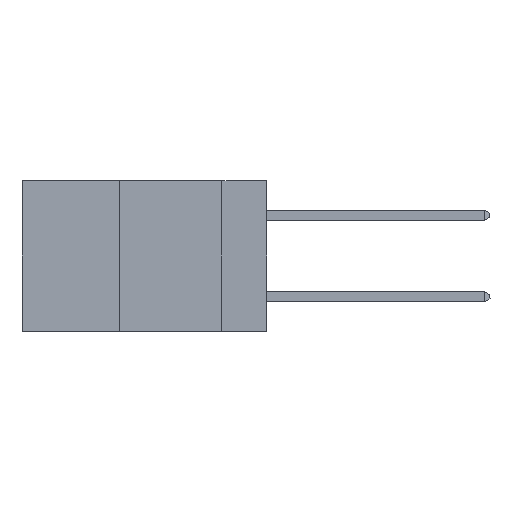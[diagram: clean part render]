
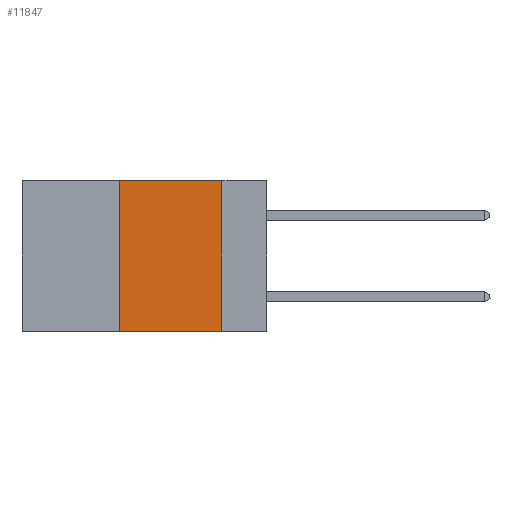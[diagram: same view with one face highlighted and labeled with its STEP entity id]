
A CAD part, left-side view. The second image highlights one B-rep face of the part: STEP entity #11847.
In plain terms, the highlighted planar face has unit normal (-1, 0, 0).
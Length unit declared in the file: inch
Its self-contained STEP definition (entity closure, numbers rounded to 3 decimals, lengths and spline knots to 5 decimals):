
#22 = EDGE_CURVE ( 'NONE', #6171, #15439, #13116, .T. ) ;
#527 = CARTESIAN_POINT ( 'NONE',  ( 0., 0.6, 0. ) ) ;
#677 = VECTOR ( 'NONE', #1669, 39.37008 ) ;
#1466 = DIRECTION ( 'NONE',  ( 1., 0., 0. ) ) ;
#1669 = DIRECTION ( 'NONE',  ( 0., -1., 0. ) ) ;
#1862 = AXIS2_PLACEMENT_3D ( 'NONE', #12660, #1466, #11447 ) ;
#2113 = LINE ( 'NONE', #4818, #7542 ) ;
#3150 = EDGE_LOOP ( 'NONE', ( #13163, #9197, #14579, #9522 ) ) ;
#3250 = VECTOR ( 'NONE', #5093, 39.37008 ) ;
#4285 = EDGE_CURVE ( 'NONE', #4865, #7811, #8316, .T. ) ;
#4818 = CARTESIAN_POINT ( 'NONE',  ( 0., 0.36, 0. ) ) ;
#4865 = VERTEX_POINT ( 'NONE', #8870 ) ;
#4944 = FACE_OUTER_BOUND ( 'NONE', #3150, .T. ) ;
#5052 = EDGE_CURVE ( 'NONE', #4865, #6171, #2113, .T. ) ;
#5093 = DIRECTION ( 'NONE',  ( 0., 0., -1. ) ) ;
#5300 = DIRECTION ( 'NONE',  ( 0., -1., 0. ) ) ;
#6171 = VERTEX_POINT ( 'NONE', #6686 ) ;
#6494 = PLANE ( 'NONE',  #1862 ) ;
#6546 = LINE ( 'NONE', #15271, #3250 ) ;
#6686 = CARTESIAN_POINT ( 'NONE',  ( 0., 0.36, 0. ) ) ;
#7542 = VECTOR ( 'NONE', #14524, 39.37008 ) ;
#7811 = VERTEX_POINT ( 'NONE', #13590 ) ;
#8316 = LINE ( 'NONE', #12654, #11237 ) ;
#8870 = CARTESIAN_POINT ( 'NONE',  ( 0., 0.36, -0.37 ) ) ;
#9197 = ORIENTED_EDGE ( 'NONE', *, *, #22, .F. ) ;
#9522 = ORIENTED_EDGE ( 'NONE', *, *, #4285, .T. ) ;
#11200 = CARTESIAN_POINT ( 'NONE',  ( 0., 0.11, 0. ) ) ;
#11237 = VECTOR ( 'NONE', #5300, 39.37008 ) ;
#11447 = DIRECTION ( 'NONE',  ( 0., 0., -1. ) ) ;
#11847 = ADVANCED_FACE ( 'NONE', ( #4944 ), #6494, .F. ) ;
#12654 = CARTESIAN_POINT ( 'NONE',  ( 0., 0.6, -0.37 ) ) ;
#12660 = CARTESIAN_POINT ( 'NONE',  ( 0., 0.6, 0. ) ) ;
#13116 = LINE ( 'NONE', #527, #677 ) ;
#13163 = ORIENTED_EDGE ( 'NONE', *, *, #13205, .F. ) ;
#13205 = EDGE_CURVE ( 'NONE', #15439, #7811, #6546, .T. ) ;
#13590 = CARTESIAN_POINT ( 'NONE',  ( 0., 0.11, -0.37 ) ) ;
#14524 = DIRECTION ( 'NONE',  ( 0., 0., 1. ) ) ;
#14579 = ORIENTED_EDGE ( 'NONE', *, *, #5052, .F. ) ;
#15271 = CARTESIAN_POINT ( 'NONE',  ( 0., 0.11, 0. ) ) ;
#15439 = VERTEX_POINT ( 'NONE', #11200 ) ;
